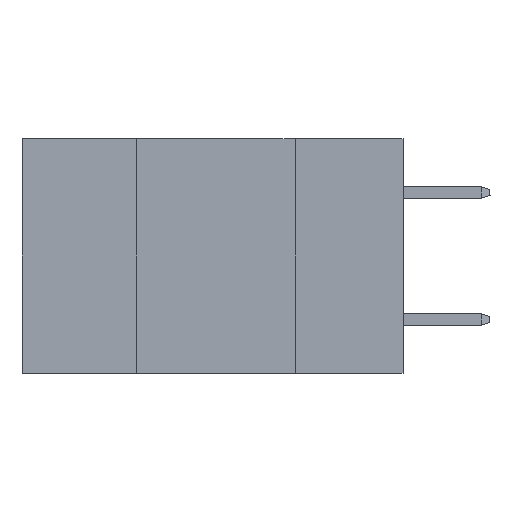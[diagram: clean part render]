
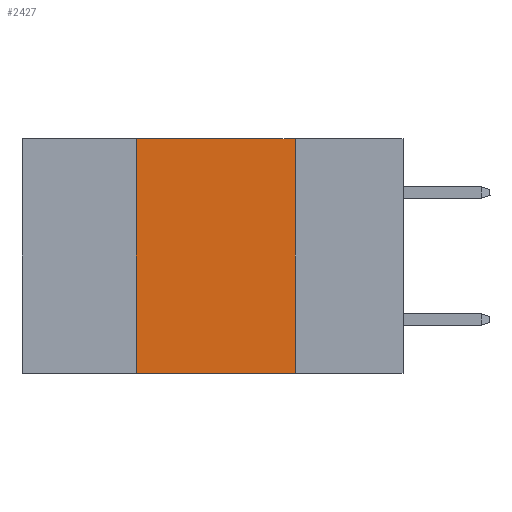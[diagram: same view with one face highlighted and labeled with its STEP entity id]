
A CAD part, left-side view. The second image highlights one B-rep face of the part: STEP entity #2427.
In plain terms, the highlighted planar face has unit normal (-1, 0, 0).
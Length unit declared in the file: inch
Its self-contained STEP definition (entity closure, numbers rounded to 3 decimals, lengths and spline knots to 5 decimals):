
#27 = ORIENTED_EDGE ( 'NONE', *, *, #21338, .F. ) ;
#141 = CARTESIAN_POINT ( 'NONE',  ( 0., 0.42, -0.37 ) ) ;
#644 = FACE_OUTER_BOUND ( 'NONE', #10077, .T. ) ;
#1206 = AXIS2_PLACEMENT_3D ( 'NONE', #17091, #28680, #5009 ) ;
#1850 = VECTOR ( 'NONE', #26504, 39.37008 ) ;
#2427 = ADVANCED_FACE ( 'NONE', ( #644 ), #19580, .F. ) ;
#4436 = ORIENTED_EDGE ( 'NONE', *, *, #19056, .T. ) ;
#4983 = CARTESIAN_POINT ( 'NONE',  ( 0., 0.42, 0. ) ) ;
#5009 = DIRECTION ( 'NONE',  ( 0., 0., -1. ) ) ;
#5638 = LINE ( 'NONE', #10572, #21060 ) ;
#6471 = VECTOR ( 'NONE', #24693, 39.37008 ) ;
#6695 = ORIENTED_EDGE ( 'NONE', *, *, #11627, .F. ) ;
#6895 = ORIENTED_EDGE ( 'NONE', *, *, #9400, .F. ) ;
#7143 = DIRECTION ( 'NONE',  ( 0., 0., 1. ) ) ;
#7586 = LINE ( 'NONE', #4983, #10808 ) ;
#7892 = CARTESIAN_POINT ( 'NONE',  ( 0., 0.6, 0. ) ) ;
#9364 = CARTESIAN_POINT ( 'NONE',  ( 0., 0.17, 0. ) ) ;
#9400 = EDGE_CURVE ( 'NONE', #25960, #27958, #7586, .T. ) ;
#10077 = EDGE_LOOP ( 'NONE', ( #6695, #27, #6895, #4436 ) ) ;
#10572 = CARTESIAN_POINT ( 'NONE',  ( 0., 0.6, -0.37 ) ) ;
#10808 = VECTOR ( 'NONE', #7143, 39.37008 ) ;
#11627 = EDGE_CURVE ( 'NONE', #12745, #15813, #29609, .T. ) ;
#12745 = VERTEX_POINT ( 'NONE', #9364 ) ;
#13195 = CARTESIAN_POINT ( 'NONE',  ( 0., 0.17, -0.37 ) ) ;
#14718 = LINE ( 'NONE', #7892, #1850 ) ;
#15813 = VERTEX_POINT ( 'NONE', #13195 ) ;
#17091 = CARTESIAN_POINT ( 'NONE',  ( 0., 0.6, 0. ) ) ;
#18549 = CARTESIAN_POINT ( 'NONE',  ( 0., 0.42, 0. ) ) ;
#19056 = EDGE_CURVE ( 'NONE', #25960, #15813, #5638, .T. ) ;
#19580 = PLANE ( 'NONE',  #1206 ) ;
#21060 = VECTOR ( 'NONE', #27156, 39.37008 ) ;
#21338 = EDGE_CURVE ( 'NONE', #27958, #12745, #14718, .T. ) ;
#24693 = DIRECTION ( 'NONE',  ( 0., 0., -1. ) ) ;
#25960 = VERTEX_POINT ( 'NONE', #141 ) ;
#26504 = DIRECTION ( 'NONE',  ( 0., -1., 0. ) ) ;
#27156 = DIRECTION ( 'NONE',  ( 0., -1., 0. ) ) ;
#27958 = VERTEX_POINT ( 'NONE', #18549 ) ;
#28680 = DIRECTION ( 'NONE',  ( 1., 0., 0. ) ) ;
#29000 = CARTESIAN_POINT ( 'NONE',  ( 0., 0.17, 0. ) ) ;
#29609 = LINE ( 'NONE', #29000, #6471 ) ;
